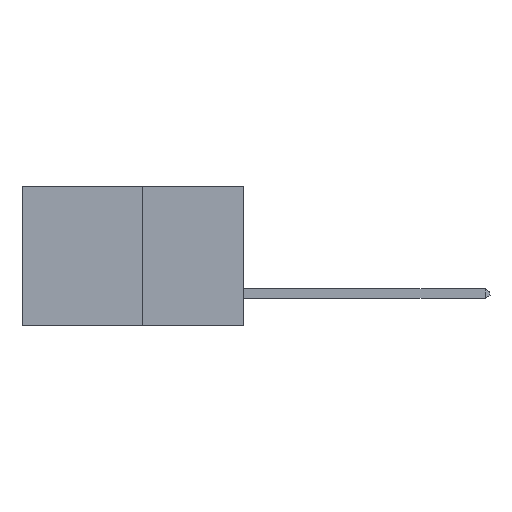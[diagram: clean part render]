
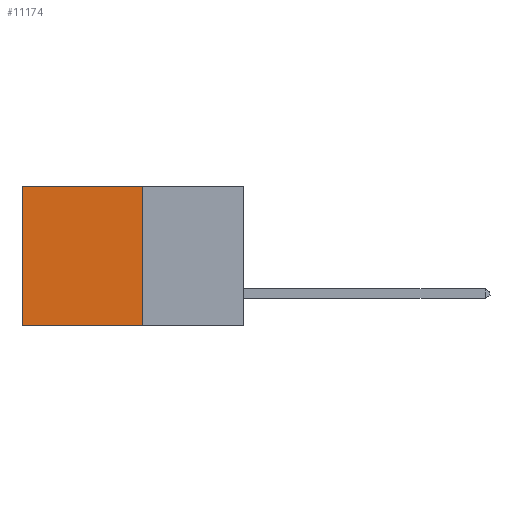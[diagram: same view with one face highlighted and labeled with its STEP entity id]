
A CAD part, left-side view. The second image highlights one B-rep face of the part: STEP entity #11174.
In plain terms, the highlighted planar face has unit normal (-1, 0, 0).
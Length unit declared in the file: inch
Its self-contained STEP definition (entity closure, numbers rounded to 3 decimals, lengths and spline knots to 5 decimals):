
#276 = VECTOR ( 'NONE', #4892, 39.37008 ) ;
#369 = ORIENTED_EDGE ( 'NONE', *, *, #4636, .F. ) ;
#372 = ORIENTED_EDGE ( 'NONE', *, *, #9171, .T. ) ;
#536 = VECTOR ( 'NONE', #599, 39.37008 ) ;
#599 = DIRECTION ( 'NONE',  ( 0., 1., 0. ) ) ;
#775 = CARTESIAN_POINT ( 'NONE',  ( 0.277, 0.27, 0. ) ) ;
#1585 = EDGE_LOOP ( 'NONE', ( #372, #2892, #369, #10681 ) ) ;
#1849 = AXIS2_PLACEMENT_3D ( 'NONE', #2638, #2672, #8750 ) ;
#2638 = CARTESIAN_POINT ( 'NONE',  ( 0.277, 0.27, -0.37 ) ) ;
#2672 = DIRECTION ( 'NONE',  ( 1., 0., 0. ) ) ;
#2739 = LINE ( 'NONE', #3127, #276 ) ;
#2828 = DIRECTION ( 'NONE',  ( 0., 0., -1. ) ) ;
#2892 = ORIENTED_EDGE ( 'NONE', *, *, #9036, .F. ) ;
#2985 = LINE ( 'NONE', #775, #536 ) ;
#3031 = CARTESIAN_POINT ( 'NONE',  ( 0.277, 0.27, -0.37 ) ) ;
#3127 = CARTESIAN_POINT ( 'NONE',  ( 0.277, 0.59, -0.37 ) ) ;
#3558 = VERTEX_POINT ( 'NONE', #9209 ) ;
#3871 = CARTESIAN_POINT ( 'NONE',  ( 0.277, 0.27, -0.37 ) ) ;
#4097 = CARTESIAN_POINT ( 'NONE',  ( 0.277, 0.27, -0.37 ) ) ;
#4416 = VECTOR ( 'NONE', #9022, 39.37008 ) ;
#4636 = EDGE_CURVE ( 'NONE', #3558, #9222, #7617, .T. ) ;
#4730 = CARTESIAN_POINT ( 'NONE',  ( 0.277, 0.59, 0. ) ) ;
#4892 = DIRECTION ( 'NONE',  ( 0., 0., -1. ) ) ;
#5025 = EDGE_CURVE ( 'NONE', #3558, #5911, #2985, .T. ) ;
#5249 = CARTESIAN_POINT ( 'NONE',  ( 0.277, 0.59, -0.37 ) ) ;
#5331 = VECTOR ( 'NONE', #2828, 39.37008 ) ;
#5911 = VERTEX_POINT ( 'NONE', #4730 ) ;
#6710 = LINE ( 'NONE', #3871, #4416 ) ;
#7617 = LINE ( 'NONE', #3031, #5331 ) ;
#7887 = PLANE ( 'NONE',  #1849 ) ;
#8657 = FACE_OUTER_BOUND ( 'NONE', #1585, .T. ) ;
#8750 = DIRECTION ( 'NONE',  ( 0., 0., -1. ) ) ;
#9022 = DIRECTION ( 'NONE',  ( 0., 1., 0. ) ) ;
#9036 = EDGE_CURVE ( 'NONE', #9222, #11139, #6710, .T. ) ;
#9171 = EDGE_CURVE ( 'NONE', #5911, #11139, #2739, .T. ) ;
#9209 = CARTESIAN_POINT ( 'NONE',  ( 0.277, 0.27, 0. ) ) ;
#9222 = VERTEX_POINT ( 'NONE', #4097 ) ;
#10681 = ORIENTED_EDGE ( 'NONE', *, *, #5025, .T. ) ;
#11139 = VERTEX_POINT ( 'NONE', #5249 ) ;
#11174 = ADVANCED_FACE ( 'NONE', ( #8657 ), #7887, .F. ) ;
